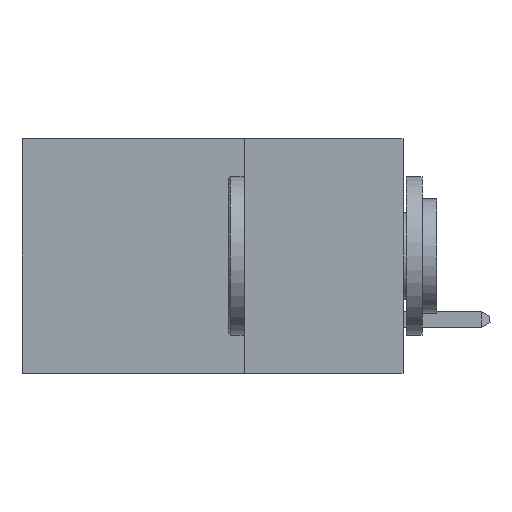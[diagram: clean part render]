
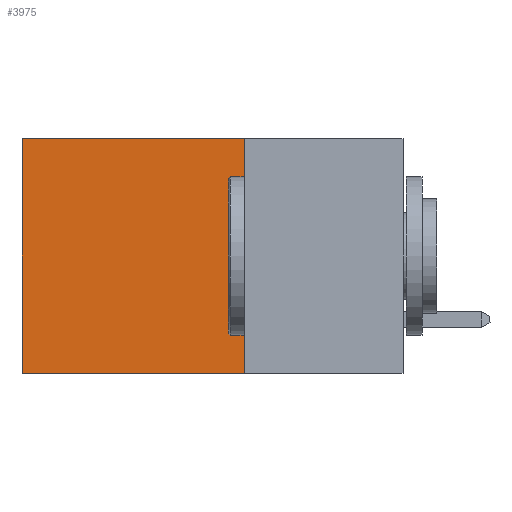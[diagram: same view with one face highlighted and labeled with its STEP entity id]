
A CAD part, left-side view. The second image highlights one B-rep face of the part: STEP entity #3975.
In plain terms, the highlighted planar face has unit normal (-1, 0, 0).
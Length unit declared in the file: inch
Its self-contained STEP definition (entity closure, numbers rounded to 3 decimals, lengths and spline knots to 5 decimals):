
#1144 = VERTEX_POINT ( 'NONE', #25951 ) ;
#1220 = EDGE_LOOP ( 'NONE', ( #33309, #23969, #24427, #14965 ) ) ;
#2589 = EDGE_CURVE ( 'NONE', #1144, #13486, #31000, .T. ) ;
#3353 = PLANE ( 'NONE',  #14060 ) ;
#3975 = ADVANCED_FACE ( 'NONE', ( #20591 ), #3353, .F. ) ;
#5514 = DIRECTION ( 'NONE',  ( 0., 0., -1. ) ) ;
#5520 = CARTESIAN_POINT ( 'NONE',  ( 0.2875, 0.6, 0. ) ) ;
#5987 = DIRECTION ( 'NONE',  ( 1., 0., 0. ) ) ;
#6522 = EDGE_CURVE ( 'NONE', #18633, #34104, #10822, .T. ) ;
#8245 = CARTESIAN_POINT ( 'NONE',  ( 0.2875, 0.6, -0.37 ) ) ;
#8811 = VECTOR ( 'NONE', #30280, 39.37008 ) ;
#9172 = CARTESIAN_POINT ( 'NONE',  ( 0.2875, 0.25, 0. ) ) ;
#10822 = LINE ( 'NONE', #5520, #24012 ) ;
#12412 = CARTESIAN_POINT ( 'NONE',  ( 0.2875, 0.25, -0.37 ) ) ;
#12601 = CARTESIAN_POINT ( 'NONE',  ( 0.2875, 0.6, 0. ) ) ;
#13486 = VERTEX_POINT ( 'NONE', #12412 ) ;
#14060 = AXIS2_PLACEMENT_3D ( 'NONE', #19039, #5987, #24400 ) ;
#14965 = ORIENTED_EDGE ( 'NONE', *, *, #29147, .T. ) ;
#15670 = DIRECTION ( 'NONE',  ( 0., 1., 0. ) ) ;
#17510 = VECTOR ( 'NONE', #15670, 39.37008 ) ;
#18633 = VERTEX_POINT ( 'NONE', #12601 ) ;
#18694 = DIRECTION ( 'NONE',  ( 0., 0., -1. ) ) ;
#19039 = CARTESIAN_POINT ( 'NONE',  ( 0.2875, 0.25, 0. ) ) ;
#20485 = EDGE_CURVE ( 'NONE', #13486, #34104, #24458, .T. ) ;
#20591 = FACE_OUTER_BOUND ( 'NONE', #1220, .T. ) ;
#23960 = VECTOR ( 'NONE', #5514, 39.37008 ) ;
#23969 = ORIENTED_EDGE ( 'NONE', *, *, #20485, .F. ) ;
#24012 = VECTOR ( 'NONE', #18694, 39.37008 ) ;
#24400 = DIRECTION ( 'NONE',  ( 0., 0., -1. ) ) ;
#24427 = ORIENTED_EDGE ( 'NONE', *, *, #2589, .F. ) ;
#24458 = LINE ( 'NONE', #26040, #17510 ) ;
#25951 = CARTESIAN_POINT ( 'NONE',  ( 0.2875, 0.25, 0. ) ) ;
#26040 = CARTESIAN_POINT ( 'NONE',  ( 0.2875, 0.25, -0.37 ) ) ;
#26419 = CARTESIAN_POINT ( 'NONE',  ( 0.2875, 0.25, 0. ) ) ;
#29147 = EDGE_CURVE ( 'NONE', #1144, #18633, #29844, .T. ) ;
#29844 = LINE ( 'NONE', #9172, #8811 ) ;
#30280 = DIRECTION ( 'NONE',  ( 0., 1., 0. ) ) ;
#31000 = LINE ( 'NONE', #26419, #23960 ) ;
#33309 = ORIENTED_EDGE ( 'NONE', *, *, #6522, .T. ) ;
#34104 = VERTEX_POINT ( 'NONE', #8245 ) ;
